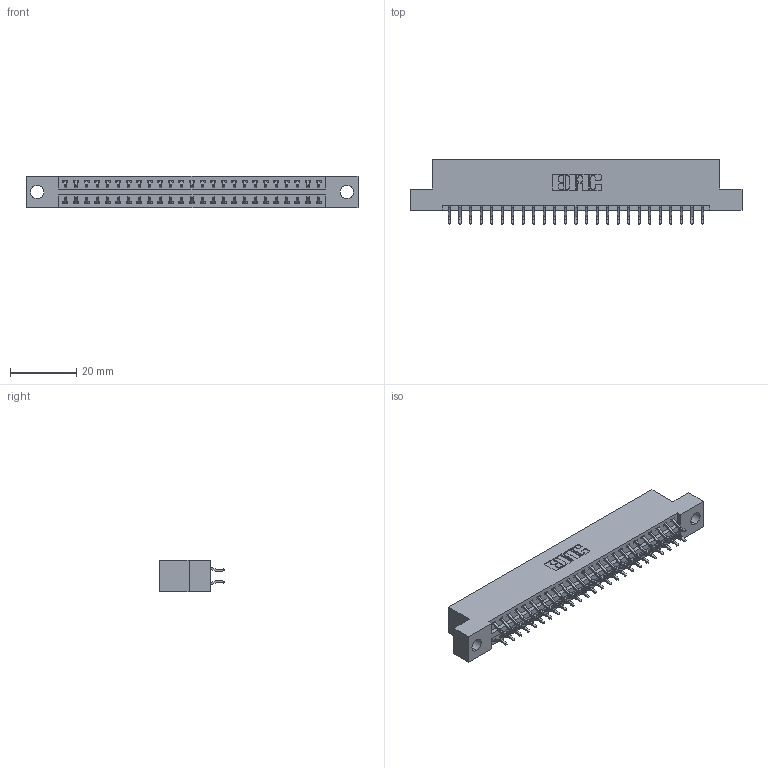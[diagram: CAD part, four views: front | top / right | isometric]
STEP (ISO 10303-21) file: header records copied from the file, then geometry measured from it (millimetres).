
FILE_DESCRIPTION (( 'STEP AP203' ), '1' );
FILE_NAME ('346-050-556-204.STEP', '2022-05-20T23:45:00', ( '' ), ( '' ), 'SwSTEP 2.0', 'SolidWorks 2020', '' );
FILE_SCHEMA (( 'CONFIG_CONTROL_DESIGN' ));
Length unit declared in the file: inch
Products named in the file (3): 346-050-556-204; 345-292-001_556 Tail; 346 Part_Flush Mounting Lugs - 0.156 Dia-TH
Assembly tree (51 placements, depth 2):
  346-050-556-204
    346 Part_Flush Mounting Lugs - 0.156 Dia-TH
    345-292-001_556 Tail  x50
Bounding box: 99.95 x 19.57 x 9.4 mm (x, y, z)
Volume: 9506.3 mm3; surface area: 12601.3 mm2
Topology: 51 solids, 51 shells, 3036 faces, 9015 edges, 5942 vertices
Faces by surface type: plane 2040, cylinder 996
Entity records: 19243 total; most frequent: CARTESIAN_POINT 3214, ORIENTED_EDGE 3134, DIRECTION 2871, EDGE_CURVE 1567, LINE 1327, VECTOR 1327, VERTEX_POINT 1042, AXIS2_PLACEMENT_3D 772
